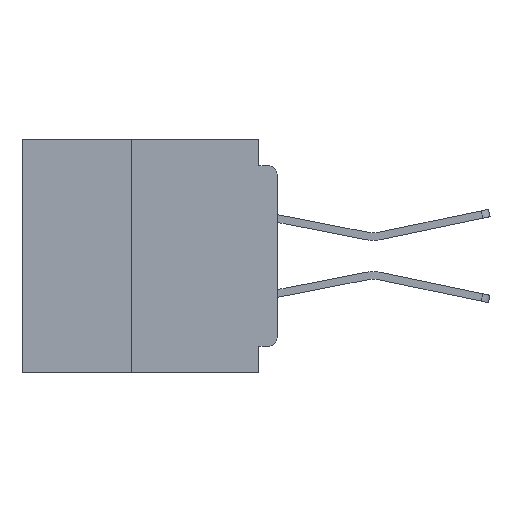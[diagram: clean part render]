
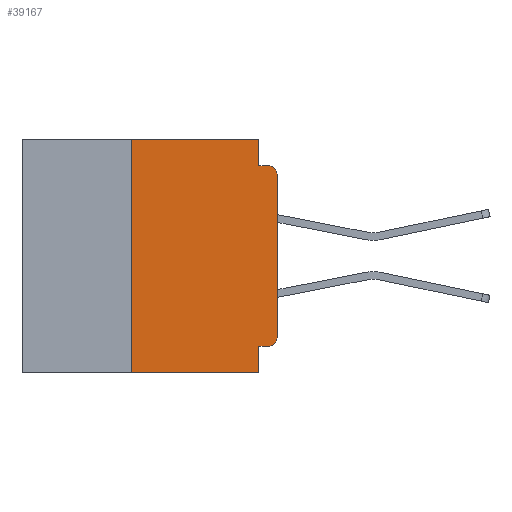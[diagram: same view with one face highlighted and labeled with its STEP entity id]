
A CAD part, left-side view. The second image highlights one B-rep face of the part: STEP entity #39167.
In plain terms, the highlighted planar face has unit normal (-1, 0, 0).
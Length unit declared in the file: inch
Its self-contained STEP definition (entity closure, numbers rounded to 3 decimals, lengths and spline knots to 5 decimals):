
#330 = DIRECTION ( 'NONE',  ( 1., 0., 0. ) ) ;
#399 = VERTEX_POINT ( 'NONE', #37508 ) ;
#479 = EDGE_LOOP ( 'NONE', ( #26600, #31307, #11469, #19091, #38330, #17679, #36661, #6895, #23854, #23896 ) ) ;
#663 = CARTESIAN_POINT ( 'NONE',  ( 0., 0.25, -0.4 ) ) ;
#798 = CARTESIAN_POINT ( 'NONE',  ( 0., 0., -0.355 ) ) ;
#1173 = VERTEX_POINT ( 'NONE', #39510 ) ;
#1973 = DIRECTION ( 'NONE',  ( 0., 0., -1. ) ) ;
#2652 = CARTESIAN_POINT ( 'NONE',  ( 0., 0.25, -0.4 ) ) ;
#2717 = VERTEX_POINT ( 'NONE', #24554 ) ;
#3363 = PLANE ( 'NONE',  #24448 ) ;
#4244 = AXIS2_PLACEMENT_3D ( 'NONE', #39232, #20726, #1973 ) ;
#4317 = LINE ( 'NONE', #25959, #27278 ) ;
#4757 = CARTESIAN_POINT ( 'NONE',  ( 0., 0.437, 0. ) ) ;
#5155 = VECTOR ( 'NONE', #7883, 39.37008 ) ;
#6895 = ORIENTED_EDGE ( 'NONE', *, *, #11084, .F. ) ;
#7229 = DIRECTION ( 'NONE',  ( 0., 0., -1. ) ) ;
#7238 = DIRECTION ( 'NONE',  ( 0., 0., 1. ) ) ;
#7420 = VERTEX_POINT ( 'NONE', #31357 ) ;
#7883 = DIRECTION ( 'NONE',  ( 0., 0., -1. ) ) ;
#7884 = DIRECTION ( 'NONE',  ( 0., -1., 0. ) ) ;
#9666 = CARTESIAN_POINT ( 'NONE',  ( 0., 0.437, 0. ) ) ;
#9835 = VECTOR ( 'NONE', #16509, 39.37008 ) ;
#10605 = VERTEX_POINT ( 'NONE', #17609 ) ;
#11084 = EDGE_CURVE ( 'NONE', #7420, #10605, #16517, .T. ) ;
#11226 = DIRECTION ( 'NONE',  ( 0., -1., 0. ) ) ;
#11347 = VERTEX_POINT ( 'NONE', #24055 ) ;
#11469 = ORIENTED_EDGE ( 'NONE', *, *, #15364, .F. ) ;
#11689 = VERTEX_POINT ( 'NONE', #663 ) ;
#12486 = EDGE_CURVE ( 'NONE', #1173, #40314, #21032, .T. ) ;
#12946 = EDGE_CURVE ( 'NONE', #40314, #36393, #4317, .T. ) ;
#13446 = LINE ( 'NONE', #798, #20749 ) ;
#13555 = VECTOR ( 'NONE', #7229, 39.37008 ) ;
#13564 = LINE ( 'NONE', #26602, #5155 ) ;
#13611 = CARTESIAN_POINT ( 'NONE',  ( 0., 0.031, -0.4 ) ) ;
#15104 = DIRECTION ( 'NONE',  ( -1., 0., 0. ) ) ;
#15364 = EDGE_CURVE ( 'NONE', #11347, #16669, #39215, .T. ) ;
#15771 = LINE ( 'NONE', #4757, #39454 ) ;
#15951 = FACE_OUTER_BOUND ( 'NONE', #479, .T. ) ;
#16509 = DIRECTION ( 'NONE',  ( 0., -1., 0. ) ) ;
#16517 = LINE ( 'NONE', #13611, #13555 ) ;
#16669 = VERTEX_POINT ( 'NONE', #33968 ) ;
#16990 = LINE ( 'NONE', #2652, #24256 ) ;
#17014 = AXIS2_PLACEMENT_3D ( 'NONE', #33654, #15104, #36737 ) ;
#17273 = EDGE_CURVE ( 'NONE', #36393, #16669, #17791, .T. ) ;
#17609 = CARTESIAN_POINT ( 'NONE',  ( 0., 0.031, -0.4 ) ) ;
#17679 = ORIENTED_EDGE ( 'NONE', *, *, #33033, .F. ) ;
#17791 = CIRCLE ( 'NONE', #17014, 0.015 ) ;
#18881 = EDGE_CURVE ( 'NONE', #2717, #399, #15771, .T. ) ;
#19091 = ORIENTED_EDGE ( 'NONE', *, *, #38116, .F. ) ;
#19167 = LINE ( 'NONE', #25699, #9835 ) ;
#20515 = CARTESIAN_POINT ( 'NONE',  ( 0., 0., -0.045 ) ) ;
#20726 = DIRECTION ( 'NONE',  ( -1., 0., 0. ) ) ;
#20749 = VECTOR ( 'NONE', #38200, 39.37008 ) ;
#21032 = CIRCLE ( 'NONE', #4244, 0.015 ) ;
#22231 = DIRECTION ( 'NONE',  ( 0., 0., -1. ) ) ;
#23627 = EDGE_CURVE ( 'NONE', #1173, #7420, #13446, .T. ) ;
#23854 = ORIENTED_EDGE ( 'NONE', *, *, #23627, .F. ) ;
#23896 = ORIENTED_EDGE ( 'NONE', *, *, #12486, .T. ) ;
#24055 = CARTESIAN_POINT ( 'NONE',  ( 0., 0.031, -0.045 ) ) ;
#24256 = VECTOR ( 'NONE', #30725, 39.37008 ) ;
#24448 = AXIS2_PLACEMENT_3D ( 'NONE', #9666, #330, #22231 ) ;
#24554 = CARTESIAN_POINT ( 'NONE',  ( 0., 0.25, 0. ) ) ;
#25699 = CARTESIAN_POINT ( 'NONE',  ( 0., 0.437, -0.4 ) ) ;
#25959 = CARTESIAN_POINT ( 'NONE',  ( 0., 0., 0. ) ) ;
#26600 = ORIENTED_EDGE ( 'NONE', *, *, #12946, .T. ) ;
#26602 = CARTESIAN_POINT ( 'NONE',  ( 0., 0.031, 0. ) ) ;
#26728 = CARTESIAN_POINT ( 'NONE',  ( 0., 0., -0.34 ) ) ;
#27278 = VECTOR ( 'NONE', #7238, 39.37008 ) ;
#29259 = EDGE_CURVE ( 'NONE', #11689, #10605, #19167, .T. ) ;
#30725 = DIRECTION ( 'NONE',  ( 0., 0., 1. ) ) ;
#31016 = VECTOR ( 'NONE', #11226, 39.37008 ) ;
#31307 = ORIENTED_EDGE ( 'NONE', *, *, #17273, .T. ) ;
#31357 = CARTESIAN_POINT ( 'NONE',  ( 0., 0.031, -0.355 ) ) ;
#31896 = CARTESIAN_POINT ( 'NONE',  ( 0., 0., -0.06 ) ) ;
#33033 = EDGE_CURVE ( 'NONE', #11689, #2717, #16990, .T. ) ;
#33654 = CARTESIAN_POINT ( 'NONE',  ( 0., 0.015, -0.06 ) ) ;
#33968 = CARTESIAN_POINT ( 'NONE',  ( 0., 0.015, -0.045 ) ) ;
#36393 = VERTEX_POINT ( 'NONE', #31896 ) ;
#36661 = ORIENTED_EDGE ( 'NONE', *, *, #29259, .T. ) ;
#36737 = DIRECTION ( 'NONE',  ( 0., 0., -1. ) ) ;
#37508 = CARTESIAN_POINT ( 'NONE',  ( 0., 0.031, 0. ) ) ;
#38116 = EDGE_CURVE ( 'NONE', #399, #11347, #13564, .T. ) ;
#38200 = DIRECTION ( 'NONE',  ( 0., 1., 0. ) ) ;
#38330 = ORIENTED_EDGE ( 'NONE', *, *, #18881, .F. ) ;
#39167 = ADVANCED_FACE ( 'NONE', ( #15951 ), #3363, .F. ) ;
#39215 = LINE ( 'NONE', #20515, #31016 ) ;
#39232 = CARTESIAN_POINT ( 'NONE',  ( 0., 0.015, -0.34 ) ) ;
#39454 = VECTOR ( 'NONE', #7884, 39.37008 ) ;
#39510 = CARTESIAN_POINT ( 'NONE',  ( 0., 0.015, -0.355 ) ) ;
#40314 = VERTEX_POINT ( 'NONE', #26728 ) ;
